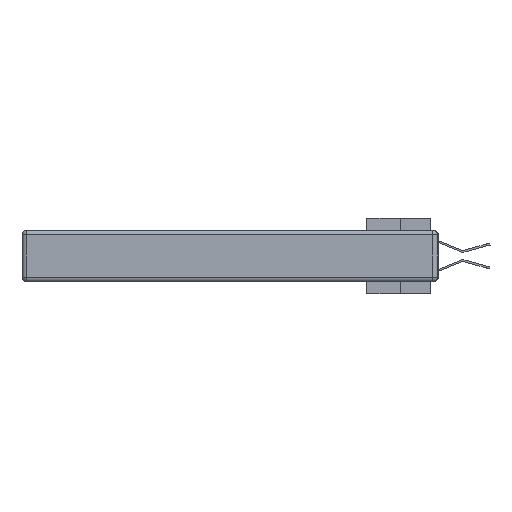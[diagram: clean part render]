
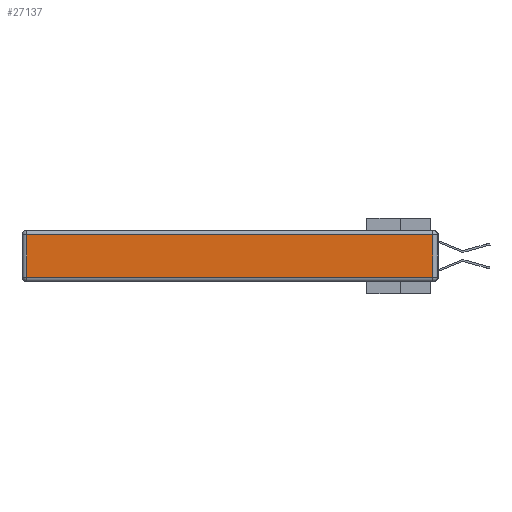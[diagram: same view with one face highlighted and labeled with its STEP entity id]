
A CAD part, left-side view. The second image highlights one B-rep face of the part: STEP entity #27137.
In plain terms, the highlighted planar face has unit normal (-1, 0, 0).
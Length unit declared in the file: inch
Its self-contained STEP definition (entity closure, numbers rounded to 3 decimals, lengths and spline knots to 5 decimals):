
#3302 = VERTEX_POINT ( 'NONE', #10895 ) ;
#4741 = LINE ( 'NONE', #19315, #22529 ) ;
#5366 = ORIENTED_EDGE ( 'NONE', *, *, #36720, .T. ) ;
#5487 = FACE_OUTER_BOUND ( 'NONE', #11668, .T. ) ;
#5997 = VECTOR ( 'NONE', #17911, 39.37008 ) ;
#6660 = CARTESIAN_POINT ( 'NONE',  ( 0., 0.03, -0.03 ) ) ;
#8490 = VECTOR ( 'NONE', #15470, 39.37008 ) ;
#9813 = AXIS2_PLACEMENT_3D ( 'NONE', #10869, #36624, #20845 ) ;
#10869 = CARTESIAN_POINT ( 'NONE',  ( 0., 0., -0.343 ) ) ;
#10895 = CARTESIAN_POINT ( 'NONE',  ( 0., 0.03, -0.313 ) ) ;
#11558 = CARTESIAN_POINT ( 'NONE',  ( 0., 0.03, -0.343 ) ) ;
#11668 = EDGE_LOOP ( 'NONE', ( #5366, #37963, #16755, #40258 ) ) ;
#12398 = EDGE_CURVE ( 'NONE', #3302, #39156, #33242, .T. ) ;
#12464 = CARTESIAN_POINT ( 'NONE',  ( 0., 2.72, -0.03 ) ) ;
#13707 = CARTESIAN_POINT ( 'NONE',  ( 0., 2.75, -0.03 ) ) ;
#14344 = LINE ( 'NONE', #13707, #25259 ) ;
#15470 = DIRECTION ( 'NONE',  ( 0., 0., -1. ) ) ;
#16755 = ORIENTED_EDGE ( 'NONE', *, *, #26853, .T. ) ;
#16894 = VERTEX_POINT ( 'NONE', #23150 ) ;
#17203 = PLANE ( 'NONE',  #9813 ) ;
#17911 = DIRECTION ( 'NONE',  ( 0., 0., 1. ) ) ;
#19315 = CARTESIAN_POINT ( 'NONE',  ( 0., 0., -0.313 ) ) ;
#20845 = DIRECTION ( 'NONE',  ( 0., 0., 1. ) ) ;
#22480 = DIRECTION ( 'NONE',  ( 0., -1., 0. ) ) ;
#22529 = VECTOR ( 'NONE', #22480, 39.37008 ) ;
#23150 = CARTESIAN_POINT ( 'NONE',  ( 0., 2.72, -0.313 ) ) ;
#25259 = VECTOR ( 'NONE', #29501, 39.37008 ) ;
#25369 = VERTEX_POINT ( 'NONE', #12464 ) ;
#26853 = EDGE_CURVE ( 'NONE', #39156, #25369, #14344, .T. ) ;
#27137 = ADVANCED_FACE ( 'NONE', ( #5487 ), #17203, .T. ) ;
#29501 = DIRECTION ( 'NONE',  ( 0., 1., 0. ) ) ;
#31274 = CARTESIAN_POINT ( 'NONE',  ( 0., 2.72, -0.343 ) ) ;
#33242 = LINE ( 'NONE', #11558, #5997 ) ;
#33283 = EDGE_CURVE ( 'NONE', #25369, #16894, #35261, .T. ) ;
#35261 = LINE ( 'NONE', #31274, #8490 ) ;
#36624 = DIRECTION ( 'NONE',  ( -1., 0., 0. ) ) ;
#36720 = EDGE_CURVE ( 'NONE', #16894, #3302, #4741, .T. ) ;
#37963 = ORIENTED_EDGE ( 'NONE', *, *, #12398, .T. ) ;
#39156 = VERTEX_POINT ( 'NONE', #6660 ) ;
#40258 = ORIENTED_EDGE ( 'NONE', *, *, #33283, .T. ) ;
